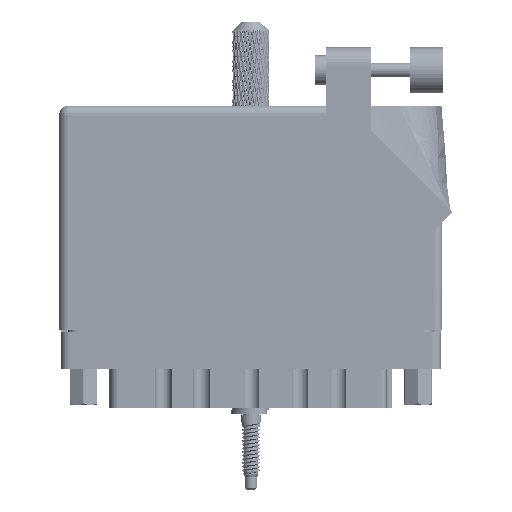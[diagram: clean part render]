
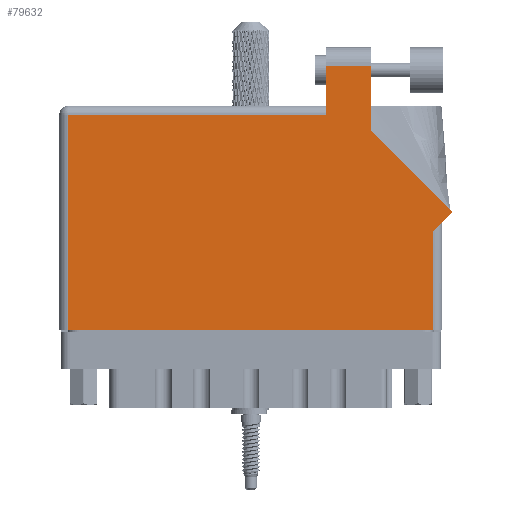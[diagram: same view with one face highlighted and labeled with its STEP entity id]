
A CAD part, front view. The second image highlights one B-rep face of the part: STEP entity #79632.
In plain terms, the highlighted face is planar.
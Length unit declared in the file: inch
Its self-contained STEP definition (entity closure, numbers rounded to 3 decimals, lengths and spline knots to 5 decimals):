
#488 = FACE_OUTER_BOUND ( 'NONE', #119279, .T. ) ;
#4910 = LINE ( 'NONE', #74938, #18975 ) ;
#6249 = VERTEX_POINT ( 'NONE', #85548 ) ;
#7804 = ORIENTED_EDGE ( 'NONE', *, *, #25007, .T. ) ;
#8008 = CARTESIAN_POINT ( 'NONE',  ( 1.819, 1.805, 0. ) ) ;
#11130 = CARTESIAN_POINT ( 'NONE',  ( 2.126, 1.36442, 0. ) ) ;
#11990 = CARTESIAN_POINT ( 'NONE',  ( 1.819, 1.805, 0. ) ) ;
#12521 = DIRECTION ( 'NONE',  ( 0.707, 0.707, 0. ) ) ;
#13265 = LINE ( 'NONE', #11990, #73049 ) ;
#16934 = AXIS2_PLACEMENT_3D ( 'NONE', #98397, #99031, #78965 ) ;
#18975 = VECTOR ( 'NONE', #93738, 39.37008 ) ;
#19555 = DIRECTION ( 'NONE',  ( 0., 1., 0. ) ) ;
#20005 = CARTESIAN_POINT ( 'NONE',  ( 0., 1.468, 0. ) ) ;
#20426 = LINE ( 'NONE', #70001, #124424 ) ;
#22239 = CARTESIAN_POINT ( 'NONE',  ( 2.612, 0.737, 0. ) ) ;
#22760 = VERTEX_POINT ( 'NONE', #58765 ) ;
#25007 = EDGE_CURVE ( 'NONE', #26708, #126434, #4910, .T. ) ;
#26708 = VERTEX_POINT ( 'NONE', #82799 ) ;
#26911 = ORIENTED_EDGE ( 'NONE', *, *, #76328, .T. ) ;
#28534 = VECTOR ( 'NONE', #76944, 39.37008 ) ;
#29014 = EDGE_CURVE ( 'NONE', #118494, #107695, #20426, .T. ) ;
#34038 = DIRECTION ( 'NONE',  ( -1., 0., 0. ) ) ;
#36371 = VECTOR ( 'NONE', #78435, 39.37008 ) ;
#37700 = ORIENTED_EDGE ( 'NONE', *, *, #112091, .T. ) ;
#39046 = ORIENTED_EDGE ( 'NONE', *, *, #90231, .T. ) ;
#39355 = EDGE_CURVE ( 'NONE', #126434, #6249, #70127, .T. ) ;
#45781 = DIRECTION ( 'NONE',  ( 0., -1., 0. ) ) ;
#51110 = DIRECTION ( 'NONE',  ( 0., -1., 0. ) ) ;
#54897 = VERTEX_POINT ( 'NONE', #71209 ) ;
#55531 = CARTESIAN_POINT ( 'NONE',  ( 0.062, 0., 0. ) ) ;
#56818 = LINE ( 'NONE', #55531, #64362 ) ;
#58765 = CARTESIAN_POINT ( 'NONE',  ( 1.819, 1.468, 0. ) ) ;
#59471 = VERTEX_POINT ( 'NONE', #85682 ) ;
#61204 = LINE ( 'NONE', #22239, #101901 ) ;
#61671 = VERTEX_POINT ( 'NONE', #8008 ) ;
#64362 = VECTOR ( 'NONE', #45781, 39.37008 ) ;
#69821 = ORIENTED_EDGE ( 'NONE', *, *, #117902, .T. ) ;
#70001 = CARTESIAN_POINT ( 'NONE',  ( 0., 0., 0. ) ) ;
#70127 = LINE ( 'NONE', #11130, #120492 ) ;
#71209 = CARTESIAN_POINT ( 'NONE',  ( 2.55, 0.675, 0. ) ) ;
#73049 = VECTOR ( 'NONE', #34038, 39.37008 ) ;
#74938 = CARTESIAN_POINT ( 'NONE',  ( 2.68271, 0.80771, 0. ) ) ;
#75651 = LINE ( 'NONE', #126761, #28534 ) ;
#76328 = EDGE_CURVE ( 'NONE', #59471, #118494, #56818, .T. ) ;
#76944 = DIRECTION ( 'NONE',  ( 0., 1., 0. ) ) ;
#77723 = CARTESIAN_POINT ( 'NONE',  ( 2.55, 0., 0. ) ) ;
#77827 = DIRECTION ( 'NONE',  ( 1., 0., 0. ) ) ;
#78435 = DIRECTION ( 'NONE',  ( -1., 0., 0. ) ) ;
#78965 = DIRECTION ( 'NONE',  ( -1., 0., 0. ) ) ;
#79600 = PLANE ( 'NONE',  #16934 ) ;
#79632 = ADVANCED_FACE ( 'NONE', ( #488 ), #79600, .F. ) ;
#82799 = CARTESIAN_POINT ( 'NONE',  ( 2.68271, 0.80771, 0. ) ) ;
#85548 = CARTESIAN_POINT ( 'NONE',  ( 2.126, 1.805, 0. ) ) ;
#85682 = CARTESIAN_POINT ( 'NONE',  ( 0.062, 1.468, 0. ) ) ;
#88344 = VECTOR ( 'NONE', #51110, 39.37008 ) ;
#89101 = CARTESIAN_POINT ( 'NONE',  ( 2.126, 1.36442, 0. ) ) ;
#90231 = EDGE_CURVE ( 'NONE', #107695, #54897, #75651, .T. ) ;
#93738 = DIRECTION ( 'NONE',  ( -0.707, 0.707, 0. ) ) ;
#94726 = ORIENTED_EDGE ( 'NONE', *, *, #29014, .T. ) ;
#98397 = CARTESIAN_POINT ( 'NONE',  ( 0., 1.53, 0. ) ) ;
#99031 = DIRECTION ( 'NONE',  ( 0., 0., -1. ) ) ;
#99592 = ORIENTED_EDGE ( 'NONE', *, *, #39355, .T. ) ;
#100069 = ORIENTED_EDGE ( 'NONE', *, *, #113626, .T. ) ;
#101901 = VECTOR ( 'NONE', #12521, 39.37008 ) ;
#101999 = ORIENTED_EDGE ( 'NONE', *, *, #127147, .T. ) ;
#102407 = CARTESIAN_POINT ( 'NONE',  ( 0.062, 0., 0. ) ) ;
#107695 = VERTEX_POINT ( 'NONE', #77723 ) ;
#112091 = EDGE_CURVE ( 'NONE', #61671, #22760, #120358, .T. ) ;
#113626 = EDGE_CURVE ( 'NONE', #54897, #26708, #61204, .T. ) ;
#117902 = EDGE_CURVE ( 'NONE', #6249, #61671, #13265, .T. ) ;
#118492 = LINE ( 'NONE', #20005, #36371 ) ;
#118494 = VERTEX_POINT ( 'NONE', #102407 ) ;
#119279 = EDGE_LOOP ( 'NONE', ( #99592, #69821, #37700, #101999, #26911, #94726, #39046, #100069, #7804 ) ) ;
#120358 = LINE ( 'NONE', #125799, #88344 ) ;
#120492 = VECTOR ( 'NONE', #19555, 39.37008 ) ;
#124424 = VECTOR ( 'NONE', #77827, 39.37008 ) ;
#125799 = CARTESIAN_POINT ( 'NONE',  ( 1.819, 1.53, 0. ) ) ;
#126434 = VERTEX_POINT ( 'NONE', #89101 ) ;
#126761 = CARTESIAN_POINT ( 'NONE',  ( 2.55, 0.737, 0. ) ) ;
#127147 = EDGE_CURVE ( 'NONE', #22760, #59471, #118492, .T. ) ;
